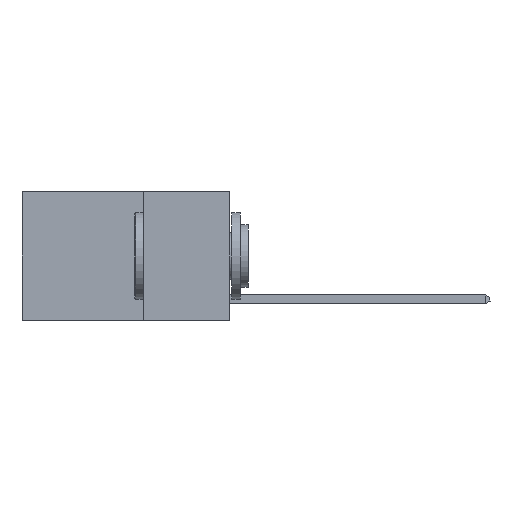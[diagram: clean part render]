
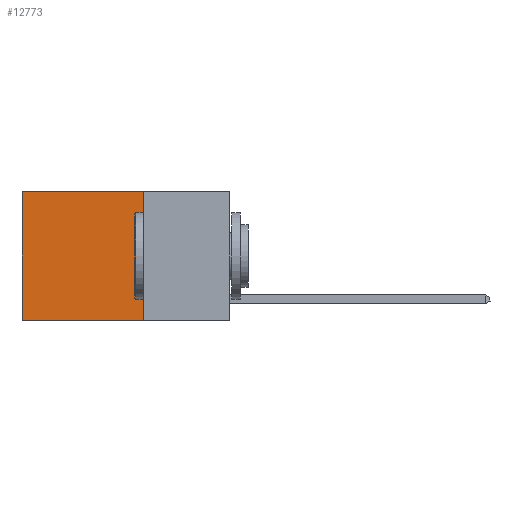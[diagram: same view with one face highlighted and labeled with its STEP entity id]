
A CAD part, left-side view. The second image highlights one B-rep face of the part: STEP entity #12773.
In plain terms, the highlighted planar face has unit normal (-1, 0, 0).
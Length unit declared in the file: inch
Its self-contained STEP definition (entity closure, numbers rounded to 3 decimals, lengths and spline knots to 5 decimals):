
#457 = LINE ( 'NONE', #7754, #5679 ) ;
#773 = EDGE_CURVE ( 'NONE', #4224, #7757, #10649, .T. ) ;
#844 = VERTEX_POINT ( 'NONE', #15934 ) ;
#1876 = DIRECTION ( 'NONE',  ( 0., 1., 0. ) ) ;
#2126 = ORIENTED_EDGE ( 'NONE', *, *, #13251, .F. ) ;
#2390 = CARTESIAN_POINT ( 'NONE',  ( 0.2625, 0.25, -0.37 ) ) ;
#2958 = CARTESIAN_POINT ( 'NONE',  ( 0.2625, 0.6, 0. ) ) ;
#3003 = DIRECTION ( 'NONE',  ( 0., 1., 0. ) ) ;
#3716 = ORIENTED_EDGE ( 'NONE', *, *, #773, .F. ) ;
#3956 = DIRECTION ( 'NONE',  ( 0., 0., -1. ) ) ;
#4030 = ORIENTED_EDGE ( 'NONE', *, *, #9178, .T. ) ;
#4203 = CARTESIAN_POINT ( 'NONE',  ( 0.2625, 0.6, 0. ) ) ;
#4224 = VERTEX_POINT ( 'NONE', #2390 ) ;
#4515 = VERTEX_POINT ( 'NONE', #2958 ) ;
#4631 = CARTESIAN_POINT ( 'NONE',  ( 0.2625, 0.6, -0.37 ) ) ;
#4761 = EDGE_LOOP ( 'NONE', ( #14123, #3716, #2126, #4030 ) ) ;
#4764 = DIRECTION ( 'NONE',  ( 0., 0., -1. ) ) ;
#5461 = LINE ( 'NONE', #4203, #10686 ) ;
#5679 = VECTOR ( 'NONE', #14045, 39.37008 ) ;
#6037 = PLANE ( 'NONE',  #9122 ) ;
#6161 = VECTOR ( 'NONE', #3003, 39.37008 ) ;
#7551 = FACE_OUTER_BOUND ( 'NONE', #4761, .T. ) ;
#7754 = CARTESIAN_POINT ( 'NONE',  ( 0.2625, 0.25, 0. ) ) ;
#7757 = VERTEX_POINT ( 'NONE', #4631 ) ;
#8258 = LINE ( 'NONE', #11772, #6161 ) ;
#8789 = CARTESIAN_POINT ( 'NONE',  ( 0.2625, 0.25, 0. ) ) ;
#9122 = AXIS2_PLACEMENT_3D ( 'NONE', #8789, #16156, #4764 ) ;
#9178 = EDGE_CURVE ( 'NONE', #844, #4515, #8258, .T. ) ;
#9841 = EDGE_CURVE ( 'NONE', #4515, #7757, #5461, .T. ) ;
#10649 = LINE ( 'NONE', #10810, #14509 ) ;
#10686 = VECTOR ( 'NONE', #3956, 39.37008 ) ;
#10810 = CARTESIAN_POINT ( 'NONE',  ( 0.2625, 0.25, -0.37 ) ) ;
#11772 = CARTESIAN_POINT ( 'NONE',  ( 0.2625, 0.25, 0. ) ) ;
#12773 = ADVANCED_FACE ( 'NONE', ( #7551 ), #6037, .F. ) ;
#13251 = EDGE_CURVE ( 'NONE', #844, #4224, #457, .T. ) ;
#14045 = DIRECTION ( 'NONE',  ( 0., 0., -1. ) ) ;
#14123 = ORIENTED_EDGE ( 'NONE', *, *, #9841, .T. ) ;
#14509 = VECTOR ( 'NONE', #1876, 39.37008 ) ;
#15934 = CARTESIAN_POINT ( 'NONE',  ( 0.2625, 0.25, 0. ) ) ;
#16156 = DIRECTION ( 'NONE',  ( 1., 0., 0. ) ) ;
